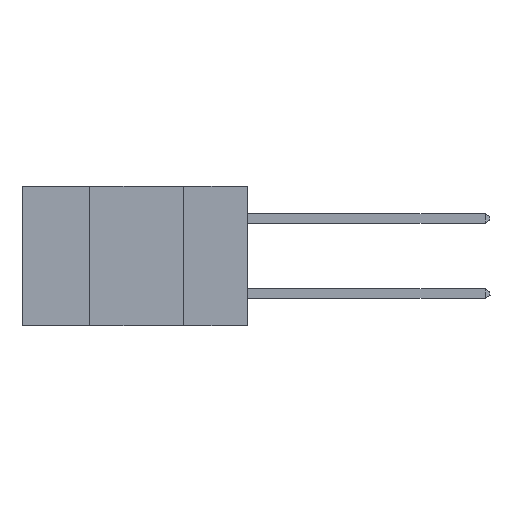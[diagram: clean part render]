
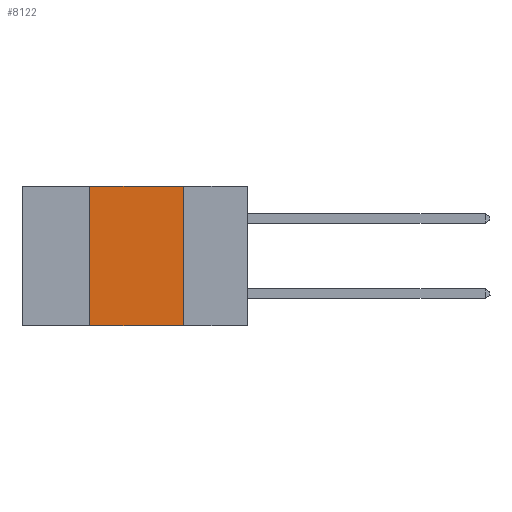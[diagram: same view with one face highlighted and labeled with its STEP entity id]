
A CAD part, left-side view. The second image highlights one B-rep face of the part: STEP entity #8122.
In plain terms, the highlighted planar face has unit normal (-1, 0, 0).
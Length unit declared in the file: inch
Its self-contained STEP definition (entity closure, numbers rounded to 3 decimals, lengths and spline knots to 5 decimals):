
#392 = VERTEX_POINT ( 'NONE', #19681 ) ;
#908 = LINE ( 'NONE', #23446, #6022 ) ;
#2470 = ORIENTED_EDGE ( 'NONE', *, *, #7300, .T. ) ;
#5214 = CARTESIAN_POINT ( 'NONE',  ( 0., 0.17, 0. ) ) ;
#5280 = EDGE_LOOP ( 'NONE', ( #18852, #21835, #21850, #2470 ) ) ;
#5662 = VECTOR ( 'NONE', #9754, 39.37008 ) ;
#6022 = VECTOR ( 'NONE', #12350, 39.37008 ) ;
#7300 = EDGE_CURVE ( 'NONE', #16532, #16598, #908, .T. ) ;
#8122 = ADVANCED_FACE ( 'NONE', ( #22892 ), #19217, .F. ) ;
#8537 = EDGE_CURVE ( 'NONE', #16532, #12746, #17748, .T. ) ;
#9754 = DIRECTION ( 'NONE',  ( 0., -1., 0. ) ) ;
#9791 = EDGE_CURVE ( 'NONE', #392, #16598, #14469, .T. ) ;
#12088 = CARTESIAN_POINT ( 'NONE',  ( 0., 0.42, 0. ) ) ;
#12214 = DIRECTION ( 'NONE',  ( 0., 0., 1. ) ) ;
#12330 = CARTESIAN_POINT ( 'NONE',  ( 0., 0.17, -0.37 ) ) ;
#12350 = DIRECTION ( 'NONE',  ( 0., -1., 0. ) ) ;
#12746 = VERTEX_POINT ( 'NONE', #22186 ) ;
#12768 = VECTOR ( 'NONE', #12214, 39.37008 ) ;
#14374 = AXIS2_PLACEMENT_3D ( 'NONE', #20357, #20673, #20636 ) ;
#14469 = LINE ( 'NONE', #5214, #23699 ) ;
#16532 = VERTEX_POINT ( 'NONE', #19601 ) ;
#16598 = VERTEX_POINT ( 'NONE', #12330 ) ;
#17748 = LINE ( 'NONE', #12088, #12768 ) ;
#18852 = ORIENTED_EDGE ( 'NONE', *, *, #9791, .F. ) ;
#19217 = PLANE ( 'NONE',  #14374 ) ;
#19601 = CARTESIAN_POINT ( 'NONE',  ( 0., 0.42, -0.37 ) ) ;
#19681 = CARTESIAN_POINT ( 'NONE',  ( 0., 0.17, 0. ) ) ;
#20022 = LINE ( 'NONE', #20920, #5662 ) ;
#20203 = DIRECTION ( 'NONE',  ( 0., 0., -1. ) ) ;
#20357 = CARTESIAN_POINT ( 'NONE',  ( 0., 0.6, 0. ) ) ;
#20636 = DIRECTION ( 'NONE',  ( 0., 0., -1. ) ) ;
#20673 = DIRECTION ( 'NONE',  ( 1., 0., 0. ) ) ;
#20920 = CARTESIAN_POINT ( 'NONE',  ( 0., 0.6, 0. ) ) ;
#21835 = ORIENTED_EDGE ( 'NONE', *, *, #22577, .F. ) ;
#21850 = ORIENTED_EDGE ( 'NONE', *, *, #8537, .F. ) ;
#22186 = CARTESIAN_POINT ( 'NONE',  ( 0., 0.42, 0. ) ) ;
#22577 = EDGE_CURVE ( 'NONE', #12746, #392, #20022, .T. ) ;
#22892 = FACE_OUTER_BOUND ( 'NONE', #5280, .T. ) ;
#23446 = CARTESIAN_POINT ( 'NONE',  ( 0., 0.6, -0.37 ) ) ;
#23699 = VECTOR ( 'NONE', #20203, 39.37008 ) ;
